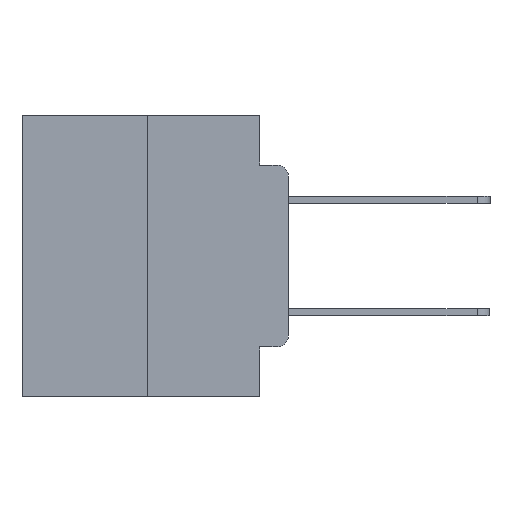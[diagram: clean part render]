
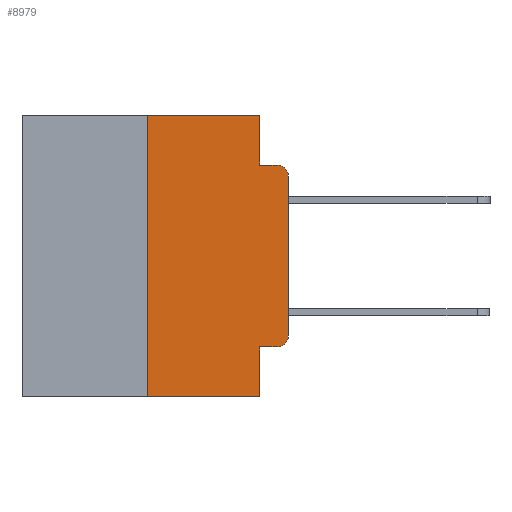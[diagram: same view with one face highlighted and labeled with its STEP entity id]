
A CAD part, left-side view. The second image highlights one B-rep face of the part: STEP entity #8979.
In plain terms, the highlighted planar face has unit normal (-1, 0, 0).
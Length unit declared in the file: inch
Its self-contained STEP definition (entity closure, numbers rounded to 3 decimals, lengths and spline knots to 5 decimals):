
#1134 = LINE ( 'NONE', #22942, #16172 ) ;
#1224 = VECTOR ( 'NONE', #11840, 39.37008 ) ;
#1279 = EDGE_CURVE ( 'NONE', #2721, #14675, #11292, .T. ) ;
#1568 = VERTEX_POINT ( 'NONE', #23573 ) ;
#2266 = EDGE_LOOP ( 'NONE', ( #3295, #3467, #3661, #3714, #3770, #3956, #4067, #4157, #4321, #4466 ) ) ;
#2457 = CARTESIAN_POINT ( 'NONE',  ( 0., 0.051, 0. ) ) ;
#2721 = VERTEX_POINT ( 'NONE', #7769 ) ;
#2817 = EDGE_CURVE ( 'NONE', #1568, #2721, #17911, .T. ) ;
#3025 = CARTESIAN_POINT ( 'NONE',  ( 0., 0.051, -0.5 ) ) ;
#3295 = ORIENTED_EDGE ( 'NONE', *, *, #16112, .T. ) ;
#3467 = ORIENTED_EDGE ( 'NONE', *, *, #14728, .T. ) ;
#3647 = CARTESIAN_POINT ( 'NONE',  ( 0., 0., -0.1085 ) ) ;
#3661 = ORIENTED_EDGE ( 'NONE', *, *, #21652, .F. ) ;
#3714 = ORIENTED_EDGE ( 'NONE', *, *, #20277, .F. ) ;
#3770 = ORIENTED_EDGE ( 'NONE', *, *, #4853, .F. ) ;
#3956 = ORIENTED_EDGE ( 'NONE', *, *, #27219, .F. ) ;
#4067 = ORIENTED_EDGE ( 'NONE', *, *, #12053, .T. ) ;
#4157 = ORIENTED_EDGE ( 'NONE', *, *, #23028, .F. ) ;
#4321 = ORIENTED_EDGE ( 'NONE', *, *, #2817, .T. ) ;
#4466 = ORIENTED_EDGE ( 'NONE', *, *, #1279, .T. ) ;
#4705 = LINE ( 'NONE', #8937, #20701 ) ;
#4713 = VERTEX_POINT ( 'NONE', #24228 ) ;
#4853 = EDGE_CURVE ( 'NONE', #12148, #19506, #4705, .T. ) ;
#6398 = DIRECTION ( 'NONE',  ( 0., 0., -1. ) ) ;
#7114 = LINE ( 'NONE', #9706, #1224 ) ;
#7198 = CARTESIAN_POINT ( 'NONE',  ( 0., 0.051, -0.4115 ) ) ;
#7341 = DIRECTION ( 'NONE',  ( 0., 0., 1. ) ) ;
#7699 = AXIS2_PLACEMENT_3D ( 'NONE', #9234, #9228, #9207 ) ;
#7769 = CARTESIAN_POINT ( 'NONE',  ( 0., 0.02, -0.4115 ) ) ;
#8170 = VERTEX_POINT ( 'NONE', #3647 ) ;
#8489 = LINE ( 'NONE', #13212, #10093 ) ;
#8869 = CARTESIAN_POINT ( 'NONE',  ( 0., 0., -0.3915 ) ) ;
#8937 = CARTESIAN_POINT ( 'NONE',  ( 0., 0.473, 0. ) ) ;
#8979 = ADVANCED_FACE ( 'NONE', ( #16561 ), #20639, .F. ) ;
#9072 = DIRECTION ( 'NONE',  ( 0., -1., 0. ) ) ;
#9184 = VECTOR ( 'NONE', #7341, 39.37008 ) ;
#9207 = DIRECTION ( 'NONE',  ( 0., 0., -1. ) ) ;
#9228 = DIRECTION ( 'NONE',  ( -1., 0., 0. ) ) ;
#9234 = CARTESIAN_POINT ( 'NONE',  ( 0., 0.02, -0.3915 ) ) ;
#9415 = DIRECTION ( 'NONE',  ( 0., 0., 1. ) ) ;
#9706 = CARTESIAN_POINT ( 'NONE',  ( 0., 0.051, -0.0885 ) ) ;
#10026 = CARTESIAN_POINT ( 'NONE',  ( 0., 0.02, -0.0885 ) ) ;
#10093 = VECTOR ( 'NONE', #9072, 39.37008 ) ;
#11069 = CARTESIAN_POINT ( 'NONE',  ( 0., 0.02, -0.1085 ) ) ;
#11292 = CIRCLE ( 'NONE', #7699, 0.02 ) ;
#11840 = DIRECTION ( 'NONE',  ( 0., -1., 0. ) ) ;
#12053 = EDGE_CURVE ( 'NONE', #12450, #15533, #8489, .T. ) ;
#12148 = VERTEX_POINT ( 'NONE', #17775 ) ;
#12368 = DIRECTION ( 'NONE',  ( 0., 0., -1. ) ) ;
#12450 = VERTEX_POINT ( 'NONE', #14481 ) ;
#13183 = DIRECTION ( 'NONE',  ( 0., 0., -1. ) ) ;
#13212 = CARTESIAN_POINT ( 'NONE',  ( 0., 0.473, -0.5 ) ) ;
#13516 = DIRECTION ( 'NONE',  ( 0., -1., 0. ) ) ;
#13550 = VECTOR ( 'NONE', #9415, 39.37008 ) ;
#14481 = CARTESIAN_POINT ( 'NONE',  ( 0., 0.25, -0.5 ) ) ;
#14621 = AXIS2_PLACEMENT_3D ( 'NONE', #11069, #25626, #13183 ) ;
#14675 = VERTEX_POINT ( 'NONE', #8869 ) ;
#14728 = EDGE_CURVE ( 'NONE', #8170, #17984, #14944, .T. ) ;
#14944 = CIRCLE ( 'NONE', #14621, 0.02 ) ;
#15533 = VERTEX_POINT ( 'NONE', #3025 ) ;
#16112 = EDGE_CURVE ( 'NONE', #14675, #8170, #18443, .T. ) ;
#16172 = VECTOR ( 'NONE', #6398, 39.37008 ) ;
#16561 = FACE_OUTER_BOUND ( 'NONE', #2266, .T. ) ;
#17775 = CARTESIAN_POINT ( 'NONE',  ( 0., 0.25, 0. ) ) ;
#17911 = LINE ( 'NONE', #7198, #22744 ) ;
#17984 = VERTEX_POINT ( 'NONE', #10026 ) ;
#18237 = LINE ( 'NONE', #2457, #23066 ) ;
#18391 = CARTESIAN_POINT ( 'NONE',  ( 0., 0.051, 0. ) ) ;
#18443 = LINE ( 'NONE', #21901, #13550 ) ;
#19357 = DIRECTION ( 'NONE',  ( 0., 0., -1. ) ) ;
#19506 = VERTEX_POINT ( 'NONE', #18391 ) ;
#19839 = CARTESIAN_POINT ( 'NONE',  ( 0., 0.25, 0. ) ) ;
#20277 = EDGE_CURVE ( 'NONE', #19506, #4713, #18237, .T. ) ;
#20639 = PLANE ( 'NONE',  #27198 ) ;
#20701 = VECTOR ( 'NONE', #13516, 39.37008 ) ;
#21352 = DIRECTION ( 'NONE',  ( 0., -1., 0. ) ) ;
#21652 = EDGE_CURVE ( 'NONE', #4713, #17984, #7114, .T. ) ;
#21901 = CARTESIAN_POINT ( 'NONE',  ( 0., 0., 0. ) ) ;
#22616 = CARTESIAN_POINT ( 'NONE',  ( 0., 0.473, 0. ) ) ;
#22744 = VECTOR ( 'NONE', #21352, 39.37008 ) ;
#22942 = CARTESIAN_POINT ( 'NONE',  ( 0., 0.051, 0. ) ) ;
#23028 = EDGE_CURVE ( 'NONE', #1568, #15533, #1134, .T. ) ;
#23066 = VECTOR ( 'NONE', #19357, 39.37008 ) ;
#23573 = CARTESIAN_POINT ( 'NONE',  ( 0., 0.051, -0.4115 ) ) ;
#24228 = CARTESIAN_POINT ( 'NONE',  ( 0., 0.051, -0.0885 ) ) ;
#24805 = DIRECTION ( 'NONE',  ( 1., 0., 0. ) ) ;
#25626 = DIRECTION ( 'NONE',  ( -1., 0., 0. ) ) ;
#25808 = LINE ( 'NONE', #19839, #9184 ) ;
#27198 = AXIS2_PLACEMENT_3D ( 'NONE', #22616, #24805, #12368 ) ;
#27219 = EDGE_CURVE ( 'NONE', #12450, #12148, #25808, .T. ) ;
